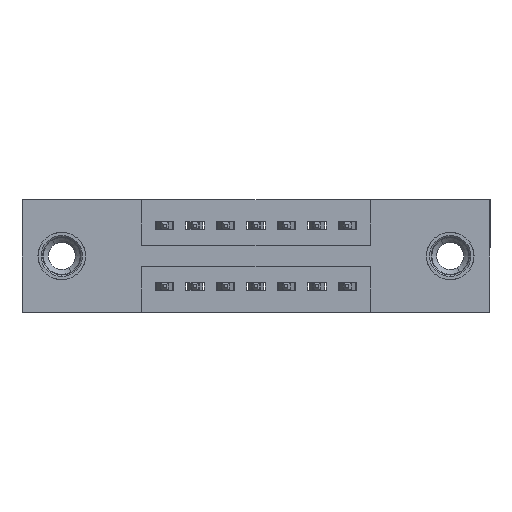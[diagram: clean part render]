
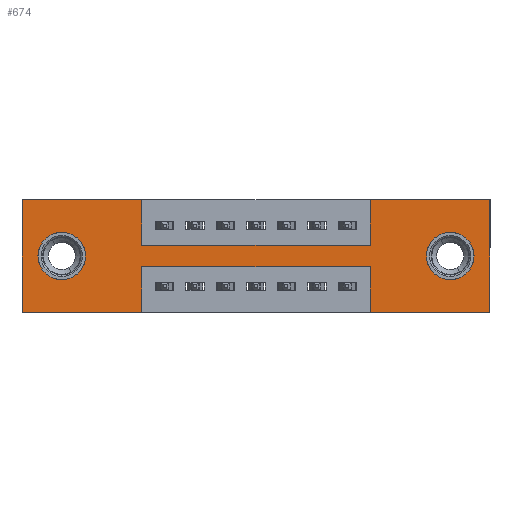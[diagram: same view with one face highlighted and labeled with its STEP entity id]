
A CAD part, front view. The second image highlights one B-rep face of the part: STEP entity #674.
In plain terms, the highlighted planar face has unit normal (0, -1, 0).
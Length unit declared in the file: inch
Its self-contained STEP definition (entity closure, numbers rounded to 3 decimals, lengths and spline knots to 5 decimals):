
#11 = VECTOR ( 'NONE', #8095, 39.37008 ) ;
#199 = VECTOR ( 'NONE', #9573, 39.37008 ) ;
#376 = LINE ( 'NONE', #12141, #10299 ) ;
#605 = DIRECTION ( 'NONE',  ( 0., 0., 1. ) ) ;
#674 = ADVANCED_FACE ( 'NONE', ( #12042, #4524, #11759 ), #2354, .T. ) ;
#750 = AXIS2_PLACEMENT_3D ( 'NONE', #1022, #7761, #2038 ) ;
#795 = EDGE_CURVE ( 'NONE', #9740, #5875, #376, .T. ) ;
#804 = CARTESIAN_POINT ( 'NONE',  ( 1.405, 0., -0.185 ) ) ;
#811 = EDGE_CURVE ( 'NONE', #1481, #11522, #5257, .T. ) ;
#856 = VERTEX_POINT ( 'NONE', #1798 ) ;
#1022 = CARTESIAN_POINT ( 'NONE',  ( 0.13, 0., -0.185 ) ) ;
#1047 = EDGE_CURVE ( 'NONE', #5875, #5118, #5399, .T. ) ;
#1187 = LINE ( 'NONE', #7368, #6029 ) ;
#1398 = CARTESIAN_POINT ( 'NONE',  ( 0., 0., -0.37 ) ) ;
#1437 = ORIENTED_EDGE ( 'NONE', *, *, #12334, .T. ) ;
#1481 = VERTEX_POINT ( 'NONE', #8812 ) ;
#1645 = EDGE_CURVE ( 'NONE', #5118, #856, #8937, .T. ) ;
#1687 = EDGE_CURVE ( 'NONE', #8912, #1878, #8645, .T. ) ;
#1798 = CARTESIAN_POINT ( 'NONE',  ( 1.1425, 0., -0.15 ) ) ;
#1831 = DIRECTION ( 'NONE',  ( 0., 0., -1. ) ) ;
#1847 = ORIENTED_EDGE ( 'NONE', *, *, #2153, .F. ) ;
#1878 = VERTEX_POINT ( 'NONE', #4594 ) ;
#1880 = CARTESIAN_POINT ( 'NONE',  ( 0.3925, 0., -0.22 ) ) ;
#2038 = DIRECTION ( 'NONE',  ( 0., 0., 1. ) ) ;
#2058 = ORIENTED_EDGE ( 'NONE', *, *, #1645, .F. ) ;
#2139 = CARTESIAN_POINT ( 'NONE',  ( 1.535, 0., -0.37 ) ) ;
#2153 = EDGE_CURVE ( 'NONE', #3749, #9740, #5748, .T. ) ;
#2296 = CARTESIAN_POINT ( 'NONE',  ( 0.13, 0., -0.107 ) ) ;
#2354 = PLANE ( 'NONE',  #8583 ) ;
#2401 = CARTESIAN_POINT ( 'NONE',  ( 0., 0., -0.37 ) ) ;
#2419 = DIRECTION ( 'NONE',  ( 0., 0., -1. ) ) ;
#2705 = EDGE_CURVE ( 'NONE', #10914, #11003, #12356, .T. ) ;
#2724 = DIRECTION ( 'NONE',  ( 1., 0., 0. ) ) ;
#2737 = DIRECTION ( 'NONE',  ( -1., 0., 0. ) ) ;
#2817 = DIRECTION ( 'NONE',  ( 0., 1., 0. ) ) ;
#2825 = ORIENTED_EDGE ( 'NONE', *, *, #11307, .F. ) ;
#3140 = ORIENTED_EDGE ( 'NONE', *, *, #795, .F. ) ;
#3189 = CARTESIAN_POINT ( 'NONE',  ( 0., 0., -0.37 ) ) ;
#3208 = LINE ( 'NONE', #7454, #5427 ) ;
#3559 = CARTESIAN_POINT ( 'NONE',  ( 1.1425, 0., -0.22 ) ) ;
#3609 = ORIENTED_EDGE ( 'NONE', *, *, #6983, .T. ) ;
#3749 = VERTEX_POINT ( 'NONE', #3189 ) ;
#3895 = EDGE_LOOP ( 'NONE', ( #6087, #3609 ) ) ;
#4052 = AXIS2_PLACEMENT_3D ( 'NONE', #12336, #7620, #10881 ) ;
#4108 = EDGE_CURVE ( 'NONE', #10647, #10966, #6145, .T. ) ;
#4479 = CARTESIAN_POINT ( 'NONE',  ( 1.1425, 0., -0.37 ) ) ;
#4524 = FACE_BOUND ( 'NONE', #3895, .T. ) ;
#4594 = CARTESIAN_POINT ( 'NONE',  ( 1.405, 0., -0.107 ) ) ;
#4693 = CARTESIAN_POINT ( 'NONE',  ( 0., 0., 0. ) ) ;
#4729 = DIRECTION ( 'NONE',  ( 0., 0., 1. ) ) ;
#4764 = CARTESIAN_POINT ( 'NONE',  ( 1.535, 0., 0. ) ) ;
#4866 = VERTEX_POINT ( 'NONE', #4951 ) ;
#4918 = EDGE_LOOP ( 'NONE', ( #11530, #11150, #12312, #2825, #8267, #10913, #10224, #2058, #6508, #3140, #1847, #5716 ) ) ;
#4939 = CARTESIAN_POINT ( 'NONE',  ( 0., 0., 0. ) ) ;
#4951 = CARTESIAN_POINT ( 'NONE',  ( 0.13, 0., -0.263 ) ) ;
#4954 = CARTESIAN_POINT ( 'NONE',  ( 0.3925, 0., -0.22 ) ) ;
#5114 = CARTESIAN_POINT ( 'NONE',  ( 0.3925, 0., -0.37 ) ) ;
#5118 = VERTEX_POINT ( 'NONE', #5273 ) ;
#5226 = LINE ( 'NONE', #1398, #11 ) ;
#5257 = LINE ( 'NONE', #4479, #7782 ) ;
#5273 = CARTESIAN_POINT ( 'NONE',  ( 0.3925, 0., -0.15 ) ) ;
#5326 = EDGE_CURVE ( 'NONE', #7144, #4866, #10568, .T. ) ;
#5371 = DIRECTION ( 'NONE',  ( -1., 0., 0. ) ) ;
#5399 = LINE ( 'NONE', #9743, #199 ) ;
#5427 = VECTOR ( 'NONE', #2724, 39.37008 ) ;
#5448 = VECTOR ( 'NONE', #4729, 39.37008 ) ;
#5716 = ORIENTED_EDGE ( 'NONE', *, *, #12093, .F. ) ;
#5748 = LINE ( 'NONE', #4693, #5448 ) ;
#5783 = DIRECTION ( 'NONE',  ( 0., -1., 0. ) ) ;
#5806 = EDGE_LOOP ( 'NONE', ( #1437, #7526 ) ) ;
#5875 = VERTEX_POINT ( 'NONE', #10181 ) ;
#6029 = VECTOR ( 'NONE', #605, 39.37008 ) ;
#6087 = ORIENTED_EDGE ( 'NONE', *, *, #5326, .T. ) ;
#6090 = EDGE_CURVE ( 'NONE', #11522, #10914, #7597, .T. ) ;
#6145 = LINE ( 'NONE', #4764, #10878 ) ;
#6423 = VECTOR ( 'NONE', #12047, 39.37008 ) ;
#6508 = ORIENTED_EDGE ( 'NONE', *, *, #1047, .F. ) ;
#6875 = VECTOR ( 'NONE', #2737, 39.37008 ) ;
#6972 = DIRECTION ( 'NONE',  ( 0., 0., -1. ) ) ;
#6983 = EDGE_CURVE ( 'NONE', #4866, #7144, #11700, .T. ) ;
#7144 = VERTEX_POINT ( 'NONE', #2296 ) ;
#7363 = VECTOR ( 'NONE', #6972, 39.37008 ) ;
#7368 = CARTESIAN_POINT ( 'NONE',  ( 1.1425, 0., 0. ) ) ;
#7371 = AXIS2_PLACEMENT_3D ( 'NONE', #8487, #2817, #9438 ) ;
#7454 = CARTESIAN_POINT ( 'NONE',  ( 0., 0., 0. ) ) ;
#7526 = ORIENTED_EDGE ( 'NONE', *, *, #1687, .T. ) ;
#7554 = DIRECTION ( 'NONE',  ( 0., 1., 0. ) ) ;
#7597 = LINE ( 'NONE', #1880, #12285 ) ;
#7620 = DIRECTION ( 'NONE',  ( 0., 1., 0. ) ) ;
#7761 = DIRECTION ( 'NONE',  ( 0., 1., 0. ) ) ;
#7782 = VECTOR ( 'NONE', #10154, 39.37008 ) ;
#8054 = AXIS2_PLACEMENT_3D ( 'NONE', #804, #7554, #1831 ) ;
#8095 = DIRECTION ( 'NONE',  ( -1., 0., 0. ) ) ;
#8188 = CARTESIAN_POINT ( 'NONE',  ( 0.3925, 0., -0.37 ) ) ;
#8212 = VERTEX_POINT ( 'NONE', #8562 ) ;
#8267 = ORIENTED_EDGE ( 'NONE', *, *, #4108, .F. ) ;
#8487 = CARTESIAN_POINT ( 'NONE',  ( 0.13, 0., -0.185 ) ) ;
#8562 = CARTESIAN_POINT ( 'NONE',  ( 1.1425, 0., 0. ) ) ;
#8583 = AXIS2_PLACEMENT_3D ( 'NONE', #2401, #5783, #2419 ) ;
#8645 = CIRCLE ( 'NONE', #4052, 0.078 ) ;
#8812 = CARTESIAN_POINT ( 'NONE',  ( 1.1425, 0., -0.37 ) ) ;
#8912 = VERTEX_POINT ( 'NONE', #10608 ) ;
#8937 = LINE ( 'NONE', #11477, #6423 ) ;
#9093 = LINE ( 'NONE', #12185, #6875 ) ;
#9251 = CARTESIAN_POINT ( 'NONE',  ( 1.535, 0., 0. ) ) ;
#9438 = DIRECTION ( 'NONE',  ( 0., 0., 1. ) ) ;
#9573 = DIRECTION ( 'NONE',  ( 0., 0., -1. ) ) ;
#9740 = VERTEX_POINT ( 'NONE', #4939 ) ;
#9743 = CARTESIAN_POINT ( 'NONE',  ( 0.3925, 0., 0. ) ) ;
#9975 = EDGE_CURVE ( 'NONE', #856, #8212, #1187, .T. ) ;
#10034 = EDGE_CURVE ( 'NONE', #8212, #10647, #3208, .T. ) ;
#10154 = DIRECTION ( 'NONE',  ( 0., 0., 1. ) ) ;
#10181 = CARTESIAN_POINT ( 'NONE',  ( 0.3925, 0., 0. ) ) ;
#10197 = DIRECTION ( 'NONE',  ( 1., 0., 0. ) ) ;
#10224 = ORIENTED_EDGE ( 'NONE', *, *, #9975, .F. ) ;
#10299 = VECTOR ( 'NONE', #10197, 39.37008 ) ;
#10475 = DIRECTION ( 'NONE',  ( 0., 0., -1. ) ) ;
#10568 = CIRCLE ( 'NONE', #7371, 0.078 ) ;
#10608 = CARTESIAN_POINT ( 'NONE',  ( 1.405, 0., -0.263 ) ) ;
#10647 = VERTEX_POINT ( 'NONE', #9251 ) ;
#10878 = VECTOR ( 'NONE', #10475, 39.37008 ) ;
#10881 = DIRECTION ( 'NONE',  ( 0., 0., -1. ) ) ;
#10913 = ORIENTED_EDGE ( 'NONE', *, *, #10034, .F. ) ;
#10914 = VERTEX_POINT ( 'NONE', #4954 ) ;
#10966 = VERTEX_POINT ( 'NONE', #2139 ) ;
#11003 = VERTEX_POINT ( 'NONE', #5114 ) ;
#11150 = ORIENTED_EDGE ( 'NONE', *, *, #6090, .F. ) ;
#11307 = EDGE_CURVE ( 'NONE', #10966, #1481, #9093, .T. ) ;
#11477 = CARTESIAN_POINT ( 'NONE',  ( 0.3925, 0., -0.15 ) ) ;
#11522 = VERTEX_POINT ( 'NONE', #3559 ) ;
#11530 = ORIENTED_EDGE ( 'NONE', *, *, #2705, .F. ) ;
#11700 = CIRCLE ( 'NONE', #750, 0.078 ) ;
#11759 = FACE_OUTER_BOUND ( 'NONE', #4918, .T. ) ;
#12042 = FACE_BOUND ( 'NONE', #5806, .T. ) ;
#12047 = DIRECTION ( 'NONE',  ( 1., 0., 0. ) ) ;
#12093 = EDGE_CURVE ( 'NONE', #11003, #3749, #5226, .T. ) ;
#12141 = CARTESIAN_POINT ( 'NONE',  ( 0., 0., 0. ) ) ;
#12185 = CARTESIAN_POINT ( 'NONE',  ( 0., 0., -0.37 ) ) ;
#12282 = CIRCLE ( 'NONE', #8054, 0.078 ) ;
#12285 = VECTOR ( 'NONE', #5371, 39.37008 ) ;
#12312 = ORIENTED_EDGE ( 'NONE', *, *, #811, .F. ) ;
#12334 = EDGE_CURVE ( 'NONE', #1878, #8912, #12282, .T. ) ;
#12336 = CARTESIAN_POINT ( 'NONE',  ( 1.405, 0., -0.185 ) ) ;
#12356 = LINE ( 'NONE', #8188, #7363 ) ;
